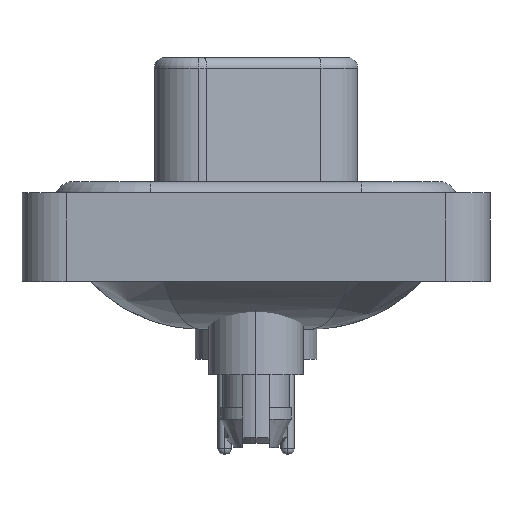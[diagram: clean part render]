
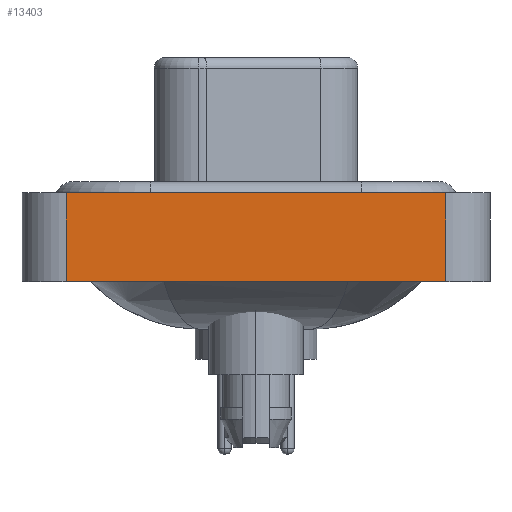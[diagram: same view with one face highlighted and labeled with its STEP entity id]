
A CAD part, left-side view. The second image highlights one B-rep face of the part: STEP entity #13403.
In plain terms, the highlighted planar face has unit normal (-1, 0, 0).
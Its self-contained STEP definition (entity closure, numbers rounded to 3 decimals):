
#140 = ORIENTED_EDGE ( 'NONE', *, *, #14789, .T. ) ;
#472 = PLANE ( 'NONE',  #4417 ) ;
#1334 = DIRECTION ( 'NONE',  ( 0., -1., 0. ) ) ;
#1395 = CARTESIAN_POINT ( 'NONE',  ( -7.3, 8.55, -3.6 ) ) ;
#2010 = FACE_OUTER_BOUND ( 'NONE', #19588, .T. ) ;
#2887 = CARTESIAN_POINT ( 'NONE',  ( -7.3, -8.55, -3.6 ) ) ;
#3457 = CARTESIAN_POINT ( 'NONE',  ( -7.3, -8.55, -3.6 ) ) ;
#4417 = AXIS2_PLACEMENT_3D ( 'NONE', #3457, #6406, #12603 ) ;
#4435 = ORIENTED_EDGE ( 'NONE', *, *, #4785, .F. ) ;
#4785 = EDGE_CURVE ( 'NONE', #12690, #13677, #17008, .T. ) ;
#4899 = EDGE_CURVE ( 'NONE', #15388, #6032, #18140, .T. ) ;
#5495 = DIRECTION ( 'NONE',  ( 0., 0., 1. ) ) ;
#6032 = VERTEX_POINT ( 'NONE', #19091 ) ;
#6045 = CARTESIAN_POINT ( 'NONE',  ( -7.3, -8.55, 0.4 ) ) ;
#6406 = DIRECTION ( 'NONE',  ( -1., 0., 0. ) ) ;
#7070 = CARTESIAN_POINT ( 'NONE',  ( -7.3, 8.55, 0.4 ) ) ;
#7153 = LINE ( 'NONE', #1395, #8270 ) ;
#7963 = VECTOR ( 'NONE', #1334, 1000. ) ;
#8270 = VECTOR ( 'NONE', #17921, 1000. ) ;
#9219 = CARTESIAN_POINT ( 'NONE',  ( -7.3, 8.55, -3.6 ) ) ;
#10315 = VECTOR ( 'NONE', #5495, 1000. ) ;
#10969 = CARTESIAN_POINT ( 'NONE',  ( -7.3, -8.55, 0.4 ) ) ;
#11199 = VECTOR ( 'NONE', #19858, 1000. ) ;
#11494 = CARTESIAN_POINT ( 'NONE',  ( -7.3, -8.55, -3.6 ) ) ;
#12603 = DIRECTION ( 'NONE',  ( 0., 0., 1. ) ) ;
#12690 = VERTEX_POINT ( 'NONE', #7070 ) ;
#13221 = LINE ( 'NONE', #11494, #10315 ) ;
#13403 = ADVANCED_FACE ( 'NONE', ( #2010 ), #472, .T. ) ;
#13677 = VERTEX_POINT ( 'NONE', #10969 ) ;
#14789 = EDGE_CURVE ( 'NONE', #6032, #13677, #13221, .T. ) ;
#15388 = VERTEX_POINT ( 'NONE', #9219 ) ;
#16251 = EDGE_CURVE ( 'NONE', #15388, #12690, #7153, .T. ) ;
#16292 = ORIENTED_EDGE ( 'NONE', *, *, #4899, .T. ) ;
#17008 = LINE ( 'NONE', #6045, #11199 ) ;
#17921 = DIRECTION ( 'NONE',  ( 0., 0., 1. ) ) ;
#18024 = ORIENTED_EDGE ( 'NONE', *, *, #16251, .F. ) ;
#18140 = LINE ( 'NONE', #2887, #7963 ) ;
#19091 = CARTESIAN_POINT ( 'NONE',  ( -7.3, -8.55, -3.6 ) ) ;
#19588 = EDGE_LOOP ( 'NONE', ( #140, #4435, #18024, #16292 ) ) ;
#19858 = DIRECTION ( 'NONE',  ( 0., -1., 0. ) ) ;
